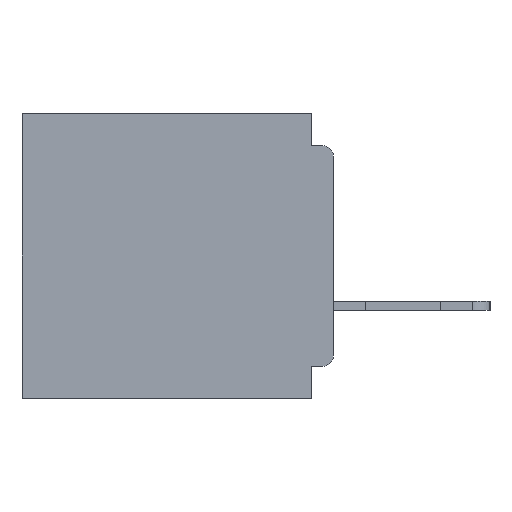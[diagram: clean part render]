
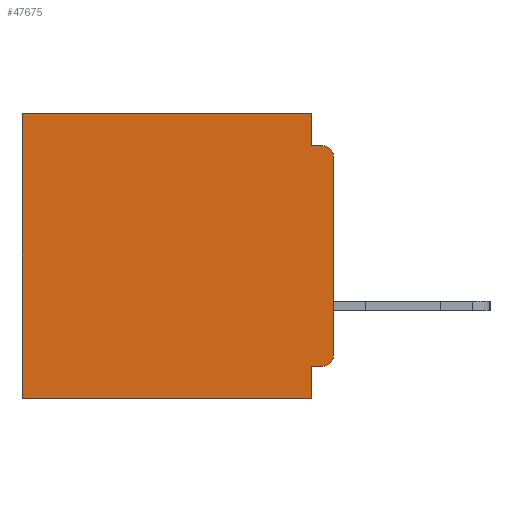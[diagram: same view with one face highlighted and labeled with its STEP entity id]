
A CAD part, left-side view. The second image highlights one B-rep face of the part: STEP entity #47675.
In plain terms, the highlighted planar face has unit normal (-1, 0, 0).
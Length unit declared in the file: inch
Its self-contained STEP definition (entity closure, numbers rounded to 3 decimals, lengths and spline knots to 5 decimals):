
#199 = ORIENTED_EDGE ( 'NONE', *, *, #34709, .T. ) ;
#584 = LINE ( 'NONE', #27769, #53463 ) ;
#1291 = DIRECTION ( 'NONE',  ( 0., 0., -1. ) ) ;
#1570 = CARTESIAN_POINT ( 'NONE',  ( 0.3, 0., -0.045 ) ) ;
#1747 = ORIENTED_EDGE ( 'NONE', *, *, #36927, .F. ) ;
#2102 = ORIENTED_EDGE ( 'NONE', *, *, #44149, .T. ) ;
#2745 = VECTOR ( 'NONE', #22893, 39.37008 ) ;
#3167 = VERTEX_POINT ( 'NONE', #24098 ) ;
#4048 = LINE ( 'NONE', #1570, #2745 ) ;
#4360 = LINE ( 'NONE', #46474, #47110 ) ;
#4792 = ORIENTED_EDGE ( 'NONE', *, *, #16642, .F. ) ;
#4970 = VERTEX_POINT ( 'NONE', #31180 ) ;
#5274 = CARTESIAN_POINT ( 'NONE',  ( 0.3, 0., -0.4 ) ) ;
#5581 = CARTESIAN_POINT ( 'NONE',  ( 0.3, 0.015, -0.355 ) ) ;
#5760 = FACE_OUTER_BOUND ( 'NONE', #50506, .T. ) ;
#5876 = CARTESIAN_POINT ( 'NONE',  ( 0.3, 0.437, 0. ) ) ;
#6044 = VERTEX_POINT ( 'NONE', #30704 ) ;
#7229 = CARTESIAN_POINT ( 'NONE',  ( 0.3, 0., 0. ) ) ;
#7642 = ORIENTED_EDGE ( 'NONE', *, *, #26754, .T. ) ;
#9475 = DIRECTION ( 'NONE',  ( 0., 0., -1. ) ) ;
#9877 = CARTESIAN_POINT ( 'NONE',  ( 0.3, 0.015, -0.045 ) ) ;
#11494 = CIRCLE ( 'NONE', #19178, 0.015 ) ;
#11738 = VERTEX_POINT ( 'NONE', #5581 ) ;
#12279 = CARTESIAN_POINT ( 'NONE',  ( 0.3, 0.031, -0.355 ) ) ;
#12361 = EDGE_CURVE ( 'NONE', #4970, #49171, #16541, .T. ) ;
#12852 = ORIENTED_EDGE ( 'NONE', *, *, #23771, .F. ) ;
#14021 = DIRECTION ( 'NONE',  ( -1., 0., 0. ) ) ;
#16541 = LINE ( 'NONE', #51451, #26608 ) ;
#16581 = DIRECTION ( 'NONE',  ( 0., 0., -1. ) ) ;
#16642 = EDGE_CURVE ( 'NONE', #31440, #44642, #4360, .T. ) ;
#17977 = DIRECTION ( 'NONE',  ( 0., 0., -1. ) ) ;
#19178 = AXIS2_PLACEMENT_3D ( 'NONE', #39612, #14021, #43908 ) ;
#19250 = LINE ( 'NONE', #43625, #27999 ) ;
#20765 = VERTEX_POINT ( 'NONE', #5876 ) ;
#20921 = VECTOR ( 'NONE', #28513, 39.37008 ) ;
#21113 = ORIENTED_EDGE ( 'NONE', *, *, #38023, .F. ) ;
#22610 = CARTESIAN_POINT ( 'NONE',  ( 0.3, 0., -0.4 ) ) ;
#22893 = DIRECTION ( 'NONE',  ( 0., -1., 0. ) ) ;
#22999 = DIRECTION ( 'NONE',  ( -1., 0., 0. ) ) ;
#23651 = ORIENTED_EDGE ( 'NONE', *, *, #12361, .F. ) ;
#23771 = EDGE_CURVE ( 'NONE', #44642, #3167, #39804, .T. ) ;
#23849 = ORIENTED_EDGE ( 'NONE', *, *, #31677, .F. ) ;
#24098 = CARTESIAN_POINT ( 'NONE',  ( 0.3, 0.437, -0.4 ) ) ;
#25809 = CIRCLE ( 'NONE', #35221, 0.015 ) ;
#26608 = VECTOR ( 'NONE', #30159, 39.37008 ) ;
#26614 = CARTESIAN_POINT ( 'NONE',  ( 0.3, 0.437, -0.4 ) ) ;
#26754 = EDGE_CURVE ( 'NONE', #4970, #36273, #11494, .T. ) ;
#26914 = DIRECTION ( 'NONE',  ( 1., 0., 0. ) ) ;
#27769 = CARTESIAN_POINT ( 'NONE',  ( 0.3, 0., -0.355 ) ) ;
#27999 = VECTOR ( 'NONE', #9475, 39.37008 ) ;
#28513 = DIRECTION ( 'NONE',  ( 0., 1., 0. ) ) ;
#29390 = VECTOR ( 'NONE', #17977, 39.37008 ) ;
#30159 = DIRECTION ( 'NONE',  ( 0., 0., -1. ) ) ;
#30704 = CARTESIAN_POINT ( 'NONE',  ( 0.3, 0.031, 0. ) ) ;
#31180 = CARTESIAN_POINT ( 'NONE',  ( 0.3, 0., -0.06 ) ) ;
#31440 = VERTEX_POINT ( 'NONE', #12279 ) ;
#31677 = EDGE_CURVE ( 'NONE', #54727, #36273, #4048, .T. ) ;
#33139 = EDGE_CURVE ( 'NONE', #20765, #3167, #52115, .T. ) ;
#33629 = LINE ( 'NONE', #7229, #20921 ) ;
#34647 = AXIS2_PLACEMENT_3D ( 'NONE', #22610, #26914, #1291 ) ;
#34709 = EDGE_CURVE ( 'NONE', #6044, #20765, #33629, .T. ) ;
#35221 = AXIS2_PLACEMENT_3D ( 'NONE', #48606, #22999, #52932 ) ;
#36209 = DIRECTION ( 'NONE',  ( 0., 1., 0. ) ) ;
#36273 = VERTEX_POINT ( 'NONE', #9877 ) ;
#36927 = EDGE_CURVE ( 'NONE', #11738, #31440, #584, .T. ) ;
#37265 = ORIENTED_EDGE ( 'NONE', *, *, #33139, .T. ) ;
#38023 = EDGE_CURVE ( 'NONE', #6044, #54727, #19250, .T. ) ;
#39612 = CARTESIAN_POINT ( 'NONE',  ( 0.3, 0.015, -0.06 ) ) ;
#39804 = LINE ( 'NONE', #5274, #51162 ) ;
#43625 = CARTESIAN_POINT ( 'NONE',  ( 0.3, 0.031, 0. ) ) ;
#43908 = DIRECTION ( 'NONE',  ( 0., 0., -1. ) ) ;
#44149 = EDGE_CURVE ( 'NONE', #11738, #49171, #25809, .T. ) ;
#44642 = VERTEX_POINT ( 'NONE', #47600 ) ;
#44856 = CARTESIAN_POINT ( 'NONE',  ( 0.3, 0., -0.34 ) ) ;
#46474 = CARTESIAN_POINT ( 'NONE',  ( 0.3, 0.031, -0.4 ) ) ;
#47110 = VECTOR ( 'NONE', #16581, 39.37008 ) ;
#47600 = CARTESIAN_POINT ( 'NONE',  ( 0.3, 0.031, -0.4 ) ) ;
#47675 = ADVANCED_FACE ( 'NONE', ( #5760 ), #48206, .F. ) ;
#48206 = PLANE ( 'NONE',  #34647 ) ;
#48606 = CARTESIAN_POINT ( 'NONE',  ( 0.3, 0.015, -0.34 ) ) ;
#48892 = CARTESIAN_POINT ( 'NONE',  ( 0.3, 0.031, -0.045 ) ) ;
#49171 = VERTEX_POINT ( 'NONE', #44856 ) ;
#50506 = EDGE_LOOP ( 'NONE', ( #23651, #7642, #23849, #21113, #199, #37265, #12852, #4792, #1747, #2102 ) ) ;
#51162 = VECTOR ( 'NONE', #52175, 39.37008 ) ;
#51451 = CARTESIAN_POINT ( 'NONE',  ( 0.3, 0., -0.4 ) ) ;
#52115 = LINE ( 'NONE', #26614, #29390 ) ;
#52175 = DIRECTION ( 'NONE',  ( 0., 1., 0. ) ) ;
#52932 = DIRECTION ( 'NONE',  ( 0., 0., -1. ) ) ;
#53463 = VECTOR ( 'NONE', #36209, 39.37008 ) ;
#54727 = VERTEX_POINT ( 'NONE', #48892 ) ;
